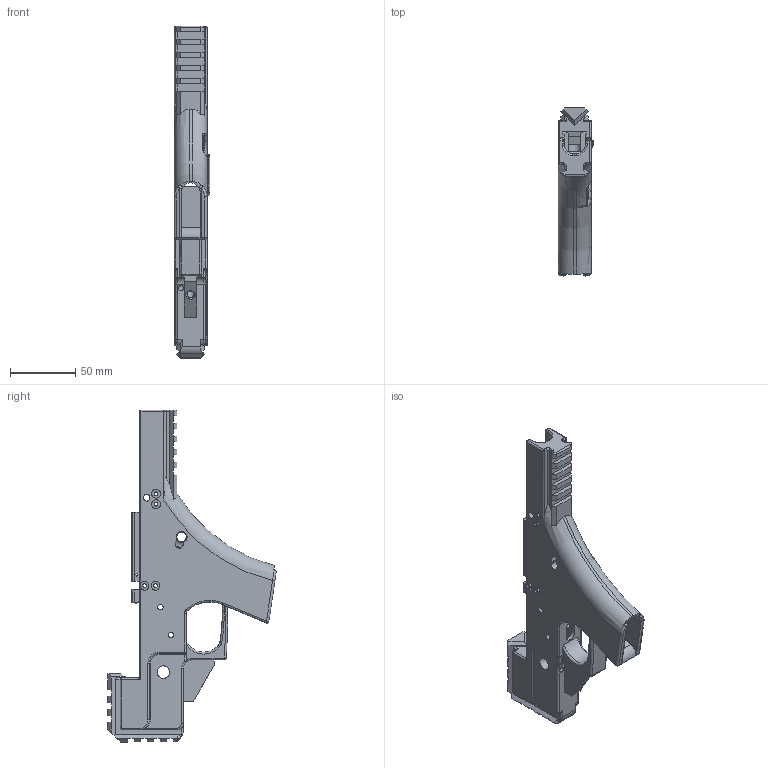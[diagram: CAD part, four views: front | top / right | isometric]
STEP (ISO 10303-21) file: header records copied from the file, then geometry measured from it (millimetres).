
FILE_DESCRIPTION(/* description */ ('RECEIVER'),/* implementation_level */ '2;1');
FILE_NAME(/* name */ '3011 Under Rail AR15 Grip Rev5 - RAMPED BARREL.stp',/* time_stamp */ '2021-08-22T23:23:24-05:00',/* author */ ('johne'),/* organization */ (''),/* preprocessor_version */ 'ST-DEVELOPER v18',/* originating_system */ 'Autodesk Inventor 2020',/* authorisation */ '');
FILE_SCHEMA (('AUTOMOTIVE_DESIGN { 1 0 10303 214 3 1 1 }'));
Length unit declared in the file: millimetre
Products named in the file (1): 3011 no rail AR15 grip RAMPED BARREL
Bounding box: 27.46 x 129.23 x 255.05 mm (x, y, z)
Volume: 209842.4 mm3; surface area: 68896.1 mm2
Topology: 1 solids, 1 shells, 496 faces, 1371 edges, 860 vertices
Faces by surface type: plane 219, cylinder 166, bspline 48, torus 48, sphere 12, cone 3
Full cylindrical faces by diameter (mm): 2.806 x1, 3 x8, 3.518 x1, 4.064 x4, 4.089 x1, 5.105 x2, 5.537 x1, 6.833 x4, 6.845 x2, 7.29 x1, 8.458 x1, 9.652 x2
Entity records: 17654 total; most frequent: CARTESIAN_POINT 5047, ORIENTED_EDGE 2714, DIRECTION 2543, EDGE_CURVE 1357, AXIS2_PLACEMENT_3D 885, VERTEX_POINT 860, LINE 773, VECTOR 773
